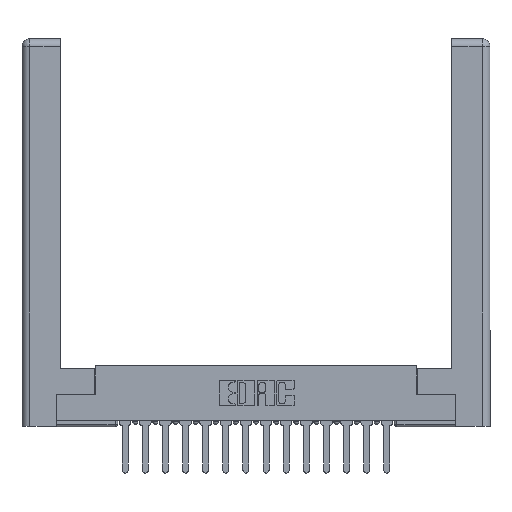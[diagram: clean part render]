
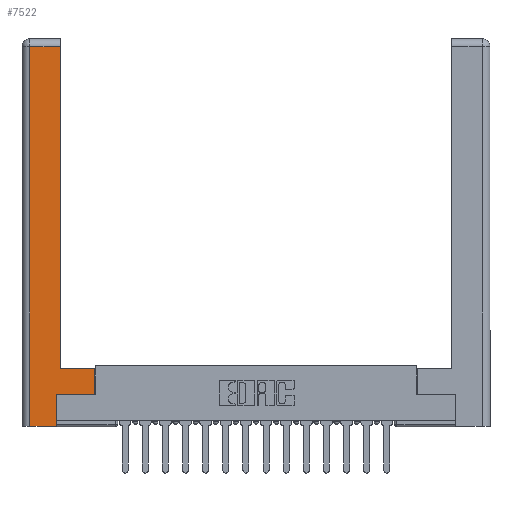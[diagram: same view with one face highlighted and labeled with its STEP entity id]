
A CAD part, top view. The second image highlights one B-rep face of the part: STEP entity #7522.
In plain terms, the highlighted planar face has unit normal (0, 0, 1).
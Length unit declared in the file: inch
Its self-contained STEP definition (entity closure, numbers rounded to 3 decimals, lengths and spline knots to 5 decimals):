
#120 = EDGE_CURVE ( 'NONE', #11565, #17851, #16531, .T. ) ;
#218 = DIRECTION ( 'NONE',  ( -1., 0., 0. ) ) ;
#323 = ORIENTED_EDGE ( 'NONE', *, *, #120, .T. ) ;
#611 = VERTEX_POINT ( 'NONE', #14974 ) ;
#946 = CARTESIAN_POINT ( 'NONE',  ( 0.0615, 2.94, 0. ) ) ;
#1224 = DIRECTION ( 'NONE',  ( 0., -1., 0. ) ) ;
#1451 = ORIENTED_EDGE ( 'NONE', *, *, #4916, .T. ) ;
#1491 = EDGE_CURVE ( 'NONE', #17851, #8507, #4105, .T. ) ;
#1665 = EDGE_CURVE ( 'NONE', #3550, #14621, #14729, .T. ) ;
#1838 = VECTOR ( 'NONE', #15488, 39.37008 ) ;
#2057 = LINE ( 'NONE', #12806, #1838 ) ;
#2368 = EDGE_LOOP ( 'NONE', ( #1451, #323, #6946, #14845, #9413, #4700, #12000, #6437 ) ) ;
#2510 = CARTESIAN_POINT ( 'NONE',  ( 0.0615, 2.94, 0. ) ) ;
#3207 = FACE_OUTER_BOUND ( 'NONE', #2368, .T. ) ;
#3325 = VECTOR ( 'NONE', #10320, 39.37008 ) ;
#3399 = VERTEX_POINT ( 'NONE', #16514 ) ;
#3550 = VERTEX_POINT ( 'NONE', #14217 ) ;
#3683 = DIRECTION ( 'NONE',  ( 1., 0., 0. ) ) ;
#3719 = EDGE_CURVE ( 'NONE', #14621, #3399, #15117, .T. ) ;
#3909 = EDGE_CURVE ( 'NONE', #611, #10239, #15340, .T. ) ;
#4105 = LINE ( 'NONE', #15238, #16060 ) ;
#4485 = CARTESIAN_POINT ( 'NONE',  ( 0.265, 0., 0. ) ) ;
#4700 = ORIENTED_EDGE ( 'NONE', *, *, #16140, .T. ) ;
#4916 = EDGE_CURVE ( 'NONE', #3399, #11565, #15304, .T. ) ;
#5052 = CARTESIAN_POINT ( 'NONE',  ( 0.565, 0.45, 0. ) ) ;
#5116 = CARTESIAN_POINT ( 'NONE',  ( 0.0615, 0., 0. ) ) ;
#5501 = VECTOR ( 'NONE', #7395, 39.37008 ) ;
#5888 = VECTOR ( 'NONE', #7835, 39.37008 ) ;
#6044 = CARTESIAN_POINT ( 'NONE',  ( 0.295, 0.45, 0. ) ) ;
#6437 = ORIENTED_EDGE ( 'NONE', *, *, #3719, .T. ) ;
#6638 = DIRECTION ( 'NONE',  ( 0., 0., -1. ) ) ;
#6745 = VECTOR ( 'NONE', #3683, 39.37008 ) ;
#6842 = EDGE_CURVE ( 'NONE', #8507, #611, #9574, .T. ) ;
#6946 = ORIENTED_EDGE ( 'NONE', *, *, #1491, .T. ) ;
#7042 = CARTESIAN_POINT ( 'NONE',  ( 0.565, 0.45, 0. ) ) ;
#7395 = DIRECTION ( 'NONE',  ( 0., 1., 0. ) ) ;
#7522 = ADVANCED_FACE ( 'NONE', ( #3207 ), #12944, .F. ) ;
#7835 = DIRECTION ( 'NONE',  ( -1., 0., 0. ) ) ;
#7907 = VECTOR ( 'NONE', #12268, 39.37008 ) ;
#8507 = VERTEX_POINT ( 'NONE', #5116 ) ;
#9250 = DIRECTION ( 'NONE',  ( 0., 1., 0. ) ) ;
#9413 = ORIENTED_EDGE ( 'NONE', *, *, #3909, .T. ) ;
#9574 = LINE ( 'NONE', #4485, #6745 ) ;
#10239 = VERTEX_POINT ( 'NONE', #13877 ) ;
#10320 = DIRECTION ( 'NONE',  ( -1., 0., 0. ) ) ;
#11415 = CARTESIAN_POINT ( 'NONE',  ( 0., 0., 0. ) ) ;
#11545 = CARTESIAN_POINT ( 'NONE',  ( 0.295, 3., 0. ) ) ;
#11565 = VERTEX_POINT ( 'NONE', #17495 ) ;
#12000 = ORIENTED_EDGE ( 'NONE', *, *, #1665, .T. ) ;
#12268 = DIRECTION ( 'NONE',  ( 0., 1., 0. ) ) ;
#12806 = CARTESIAN_POINT ( 'NONE',  ( 0.565, 0.245, 0. ) ) ;
#12944 = PLANE ( 'NONE',  #15316 ) ;
#13877 = CARTESIAN_POINT ( 'NONE',  ( 0.265, 0.245, 0. ) ) ;
#14217 = CARTESIAN_POINT ( 'NONE',  ( 0.565, 0.245, 0. ) ) ;
#14621 = VERTEX_POINT ( 'NONE', #7042 ) ;
#14729 = LINE ( 'NONE', #5052, #16265 ) ;
#14845 = ORIENTED_EDGE ( 'NONE', *, *, #6842, .T. ) ;
#14974 = CARTESIAN_POINT ( 'NONE',  ( 0.265, 0., 0. ) ) ;
#15117 = LINE ( 'NONE', #6044, #3325 ) ;
#15181 = CARTESIAN_POINT ( 'NONE',  ( 0.265, 0.245, 0. ) ) ;
#15238 = CARTESIAN_POINT ( 'NONE',  ( 0.0615, 0., 0. ) ) ;
#15304 = LINE ( 'NONE', #11545, #5501 ) ;
#15316 = AXIS2_PLACEMENT_3D ( 'NONE', #11415, #6638, #218 ) ;
#15340 = LINE ( 'NONE', #15181, #7907 ) ;
#15488 = DIRECTION ( 'NONE',  ( 1., 0., 0. ) ) ;
#16060 = VECTOR ( 'NONE', #1224, 39.37008 ) ;
#16140 = EDGE_CURVE ( 'NONE', #10239, #3550, #2057, .T. ) ;
#16265 = VECTOR ( 'NONE', #9250, 39.37008 ) ;
#16514 = CARTESIAN_POINT ( 'NONE',  ( 0.295, 0.45, 0. ) ) ;
#16531 = LINE ( 'NONE', #946, #5888 ) ;
#17495 = CARTESIAN_POINT ( 'NONE',  ( 0.295, 2.94, 0. ) ) ;
#17851 = VERTEX_POINT ( 'NONE', #2510 ) ;
